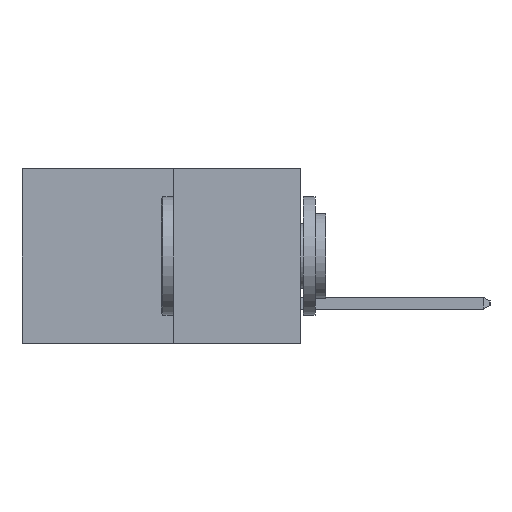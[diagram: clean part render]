
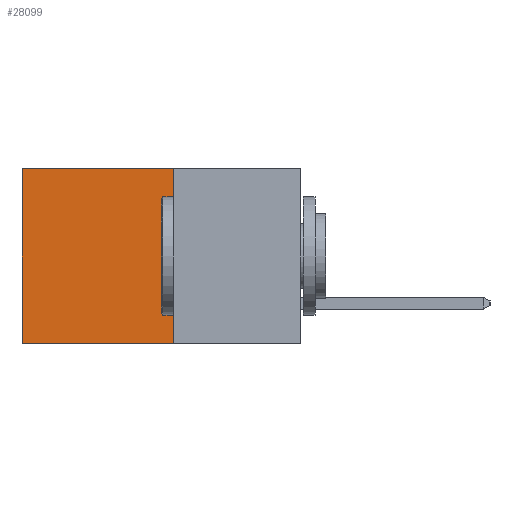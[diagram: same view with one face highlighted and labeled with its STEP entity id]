
A CAD part, left-side view. The second image highlights one B-rep face of the part: STEP entity #28099.
In plain terms, the highlighted planar face has unit normal (-1, 0, 0).
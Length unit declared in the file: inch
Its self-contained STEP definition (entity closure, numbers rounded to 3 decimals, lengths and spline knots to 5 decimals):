
#695 = DIRECTION ( 'NONE',  ( 0., 1., 0. ) ) ;
#1218 = CARTESIAN_POINT ( 'NONE',  ( 0.277, 0.27, -0.37 ) ) ;
#2135 = VECTOR ( 'NONE', #20543, 39.37008 ) ;
#3225 = EDGE_CURVE ( 'NONE', #8192, #6792, #29847, .T. ) ;
#3350 = CARTESIAN_POINT ( 'NONE',  ( 0.277, 0.27, -0.37 ) ) ;
#3656 = CARTESIAN_POINT ( 'NONE',  ( 0.277, 0.59, 0. ) ) ;
#4485 = ORIENTED_EDGE ( 'NONE', *, *, #3225, .T. ) ;
#5234 = VECTOR ( 'NONE', #24511, 39.37008 ) ;
#5739 = DIRECTION ( 'NONE',  ( 0., 0., -1. ) ) ;
#6198 = VERTEX_POINT ( 'NONE', #12229 ) ;
#6792 = VERTEX_POINT ( 'NONE', #24201 ) ;
#7409 = VECTOR ( 'NONE', #695, 39.37008 ) ;
#7462 = ORIENTED_EDGE ( 'NONE', *, *, #18507, .T. ) ;
#7620 = CARTESIAN_POINT ( 'NONE',  ( 0.277, 0.27, -0.37 ) ) ;
#8192 = VERTEX_POINT ( 'NONE', #3656 ) ;
#10564 = PLANE ( 'NONE',  #24838 ) ;
#12229 = CARTESIAN_POINT ( 'NONE',  ( 0.277, 0.27, 0. ) ) ;
#12266 = EDGE_CURVE ( 'NONE', #6198, #23566, #15795, .T. ) ;
#15795 = LINE ( 'NONE', #1218, #2135 ) ;
#17769 = EDGE_CURVE ( 'NONE', #23566, #6792, #23717, .T. ) ;
#18507 = EDGE_CURVE ( 'NONE', #6198, #8192, #26631, .T. ) ;
#20261 = DIRECTION ( 'NONE',  ( 1., 0., 0. ) ) ;
#20543 = DIRECTION ( 'NONE',  ( 0., 0., -1. ) ) ;
#21928 = ORIENTED_EDGE ( 'NONE', *, *, #17769, .F. ) ;
#22389 = EDGE_LOOP ( 'NONE', ( #4485, #21928, #30821, #7462 ) ) ;
#22571 = CARTESIAN_POINT ( 'NONE',  ( 0.277, 0.27, -0.37 ) ) ;
#23008 = FACE_OUTER_BOUND ( 'NONE', #22389, .T. ) ;
#23566 = VERTEX_POINT ( 'NONE', #22571 ) ;
#23717 = LINE ( 'NONE', #7620, #5234 ) ;
#24201 = CARTESIAN_POINT ( 'NONE',  ( 0.277, 0.59, -0.37 ) ) ;
#24511 = DIRECTION ( 'NONE',  ( 0., 1., 0. ) ) ;
#24770 = CARTESIAN_POINT ( 'NONE',  ( 0.277, 0.59, -0.37 ) ) ;
#24838 = AXIS2_PLACEMENT_3D ( 'NONE', #3350, #20261, #5739 ) ;
#25945 = DIRECTION ( 'NONE',  ( 0., 0., -1. ) ) ;
#26631 = LINE ( 'NONE', #29412, #7409 ) ;
#28099 = ADVANCED_FACE ( 'NONE', ( #23008 ), #10564, .F. ) ;
#29108 = VECTOR ( 'NONE', #25945, 39.37008 ) ;
#29412 = CARTESIAN_POINT ( 'NONE',  ( 0.277, 0.27, 0. ) ) ;
#29847 = LINE ( 'NONE', #24770, #29108 ) ;
#30821 = ORIENTED_EDGE ( 'NONE', *, *, #12266, .F. ) ;
